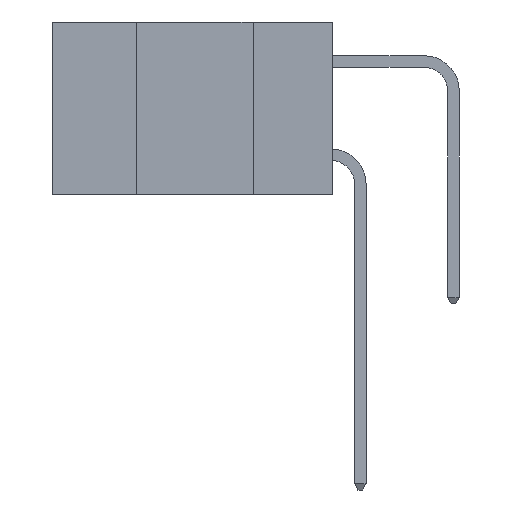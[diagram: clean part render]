
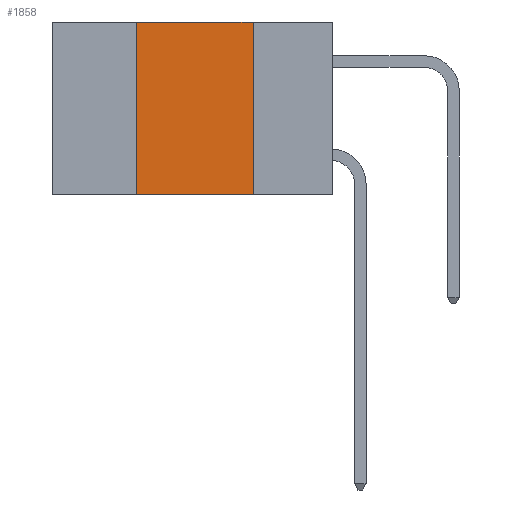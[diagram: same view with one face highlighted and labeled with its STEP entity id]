
A CAD part, left-side view. The second image highlights one B-rep face of the part: STEP entity #1858.
In plain terms, the highlighted planar face has unit normal (-1, 0, 0).
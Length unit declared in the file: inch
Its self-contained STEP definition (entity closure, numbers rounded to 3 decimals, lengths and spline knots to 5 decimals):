
#124 = CARTESIAN_POINT ( 'NONE',  ( 0., 0.42, -0.37 ) ) ;
#716 = CARTESIAN_POINT ( 'NONE',  ( 0., 0.6, 0. ) ) ;
#1096 = EDGE_LOOP ( 'NONE', ( #2805, #12856, #17657, #2355 ) ) ;
#1199 = LINE ( 'NONE', #1502, #17679 ) ;
#1297 = LINE ( 'NONE', #716, #9149 ) ;
#1502 = CARTESIAN_POINT ( 'NONE',  ( 0., 0.17, -0.37 ) ) ;
#1743 = EDGE_CURVE ( 'NONE', #2483, #17621, #1297, .T. ) ;
#1858 = ADVANCED_FACE ( 'NONE', ( #19576 ), #8054, .F. ) ;
#2355 = ORIENTED_EDGE ( 'NONE', *, *, #4158, .T. ) ;
#2483 = VERTEX_POINT ( 'NONE', #21258 ) ;
#2805 = ORIENTED_EDGE ( 'NONE', *, *, #11381, .F. ) ;
#3330 = VERTEX_POINT ( 'NONE', #124 ) ;
#4158 = EDGE_CURVE ( 'NONE', #3330, #4623, #15298, .T. ) ;
#4439 = EDGE_CURVE ( 'NONE', #3330, #2483, #4798, .T. ) ;
#4623 = VERTEX_POINT ( 'NONE', #14529 ) ;
#4798 = LINE ( 'NONE', #16519, #13011 ) ;
#6590 = DIRECTION ( 'NONE',  ( 0., 0., -1. ) ) ;
#6812 = CARTESIAN_POINT ( 'NONE',  ( 0., 0.17, 0. ) ) ;
#8054 = PLANE ( 'NONE',  #19580 ) ;
#9149 = VECTOR ( 'NONE', #11280, 39.37008 ) ;
#10964 = CARTESIAN_POINT ( 'NONE',  ( 0., 0.6, 0. ) ) ;
#11280 = DIRECTION ( 'NONE',  ( 0., -1., 0. ) ) ;
#11381 = EDGE_CURVE ( 'NONE', #17621, #4623, #1199, .T. ) ;
#11415 = DIRECTION ( 'NONE',  ( 0., 0., -1. ) ) ;
#11467 = DIRECTION ( 'NONE',  ( 1., 0., 0. ) ) ;
#12856 = ORIENTED_EDGE ( 'NONE', *, *, #1743, .F. ) ;
#13011 = VECTOR ( 'NONE', #16288, 39.37008 ) ;
#14292 = VECTOR ( 'NONE', #19508, 39.37008 ) ;
#14529 = CARTESIAN_POINT ( 'NONE',  ( 0., 0.17, -0.37 ) ) ;
#15298 = LINE ( 'NONE', #19564, #14292 ) ;
#16288 = DIRECTION ( 'NONE',  ( 0., 0., 1. ) ) ;
#16519 = CARTESIAN_POINT ( 'NONE',  ( 0., 0.42, -0.37 ) ) ;
#17621 = VERTEX_POINT ( 'NONE', #6812 ) ;
#17657 = ORIENTED_EDGE ( 'NONE', *, *, #4439, .F. ) ;
#17679 = VECTOR ( 'NONE', #6590, 39.37008 ) ;
#19508 = DIRECTION ( 'NONE',  ( 0., -1., 0. ) ) ;
#19564 = CARTESIAN_POINT ( 'NONE',  ( 0., 0.6, -0.37 ) ) ;
#19576 = FACE_OUTER_BOUND ( 'NONE', #1096, .T. ) ;
#19580 = AXIS2_PLACEMENT_3D ( 'NONE', #10964, #11467, #11415 ) ;
#21258 = CARTESIAN_POINT ( 'NONE',  ( 0., 0.42, 0. ) ) ;
